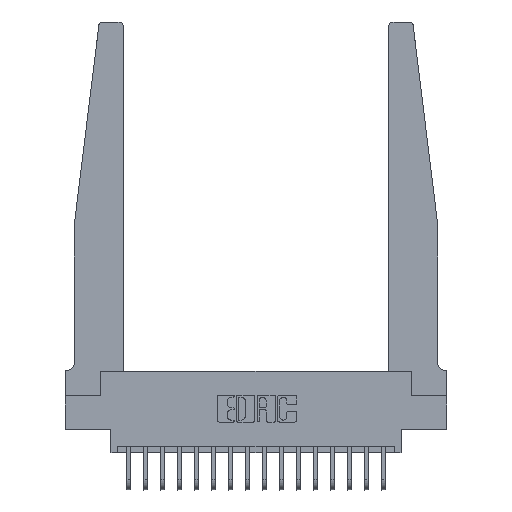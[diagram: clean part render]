
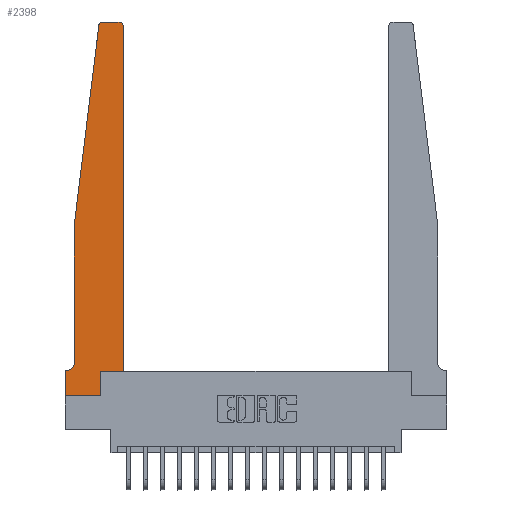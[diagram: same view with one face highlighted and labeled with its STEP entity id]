
A CAD part, top view. The second image highlights one B-rep face of the part: STEP entity #2398.
In plain terms, the highlighted planar face has unit normal (0, 0, 1).
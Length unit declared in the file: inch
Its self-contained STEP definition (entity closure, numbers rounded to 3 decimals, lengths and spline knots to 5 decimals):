
#23 = VECTOR ( 'NONE', #3496, 39.37008 ) ;
#395 = VERTEX_POINT ( 'NONE', #11442 ) ;
#416 = LINE ( 'NONE', #11971, #4247 ) ;
#700 = CARTESIAN_POINT ( 'NONE',  ( 0., 0.1875, 0.37 ) ) ;
#761 = CARTESIAN_POINT ( 'NONE',  ( 0.065, 0.2375, 0.37 ) ) ;
#1073 = AXIS2_PLACEMENT_3D ( 'NONE', #1193, #7030, #4144 ) ;
#1103 = VECTOR ( 'NONE', #1638, 39.37008 ) ;
#1130 = ORIENTED_EDGE ( 'NONE', *, *, #9392, .T. ) ;
#1193 = CARTESIAN_POINT ( 'NONE',  ( 0.395, 2.72, 0.37 ) ) ;
#1266 = VERTEX_POINT ( 'NONE', #8706 ) ;
#1410 = DIRECTION ( 'NONE',  ( 1., 0., 0. ) ) ;
#1638 = DIRECTION ( 'NONE',  ( 0., 1., 0. ) ) ;
#1659 = EDGE_CURVE ( 'NONE', #17871, #16791, #14069, .T. ) ;
#1807 = EDGE_CURVE ( 'NONE', #6830, #1266, #15064, .T. ) ;
#2285 = LINE ( 'NONE', #8151, #11412 ) ;
#2296 = FACE_OUTER_BOUND ( 'NONE', #10559, .T. ) ;
#2398 = ADVANCED_FACE ( 'NONE', ( #2296 ), #6512, .T. ) ;
#2771 = ORIENTED_EDGE ( 'NONE', *, *, #8517, .T. ) ;
#2815 = CARTESIAN_POINT ( 'NONE',  ( 0.2605, 0., 0.37 ) ) ;
#3151 = DIRECTION ( 'NONE',  ( 0., 1., 0. ) ) ;
#3366 = CARTESIAN_POINT ( 'NONE',  ( 0., 0.1875, 0.37 ) ) ;
#3496 = DIRECTION ( 'NONE',  ( 0., -1., 0. ) ) ;
#3754 = DIRECTION ( 'NONE',  ( 1., 0., 0. ) ) ;
#3782 = VECTOR ( 'NONE', #3754, 39.37008 ) ;
#3807 = ORIENTED_EDGE ( 'NONE', *, *, #1659, .T. ) ;
#3836 = VECTOR ( 'NONE', #13923, 39.37008 ) ;
#3914 = ORIENTED_EDGE ( 'NONE', *, *, #5635, .T. ) ;
#3952 = CARTESIAN_POINT ( 'NONE',  ( 0.425, 0.18, 0.37 ) ) ;
#4144 = DIRECTION ( 'NONE',  ( 1., 0., 0. ) ) ;
#4247 = VECTOR ( 'NONE', #17502, 39.37008 ) ;
#4494 = VERTEX_POINT ( 'NONE', #15113 ) ;
#4569 = CARTESIAN_POINT ( 'NONE',  ( 0.015, 0.2375, 0.37 ) ) ;
#4666 = DIRECTION ( 'NONE',  ( 0., 0., -1. ) ) ;
#4857 = CARTESIAN_POINT ( 'NONE',  ( 0.395, 2.75, 0.37 ) ) ;
#5635 = EDGE_CURVE ( 'NONE', #17623, #395, #10920, .T. ) ;
#5710 = ORIENTED_EDGE ( 'NONE', *, *, #17964, .T. ) ;
#5864 = ORIENTED_EDGE ( 'NONE', *, *, #12628, .T. ) ;
#6148 = VERTEX_POINT ( 'NONE', #17131 ) ;
#6265 = CIRCLE ( 'NONE', #1073, 0.03 ) ;
#6512 = PLANE ( 'NONE',  #12180 ) ;
#6687 = DIRECTION ( 'NONE',  ( -1., 0., 0. ) ) ;
#6830 = VERTEX_POINT ( 'NONE', #700 ) ;
#7030 = DIRECTION ( 'NONE',  ( 0., 0., 1. ) ) ;
#7727 = DIRECTION ( 'NONE',  ( -1., 0., 0. ) ) ;
#7772 = CARTESIAN_POINT ( 'NONE',  ( 0.25, 2.75, 0.37 ) ) ;
#7882 = DIRECTION ( 'NONE',  ( 0., -1., 0. ) ) ;
#8151 = CARTESIAN_POINT ( 'NONE',  ( 0.065, 0.1875, 0.37 ) ) ;
#8205 = LINE ( 'NONE', #3952, #3782 ) ;
#8338 = VERTEX_POINT ( 'NONE', #15226 ) ;
#8358 = CARTESIAN_POINT ( 'NONE',  ( 0., 0., 0.37 ) ) ;
#8517 = EDGE_CURVE ( 'NONE', #4494, #6830, #2285, .T. ) ;
#8706 = CARTESIAN_POINT ( 'NONE',  ( 0., 0., 0.37 ) ) ;
#8928 = LINE ( 'NONE', #10393, #15986 ) ;
#9020 = CARTESIAN_POINT ( 'NONE',  ( 0.425, 0.18, 0.37 ) ) ;
#9392 = EDGE_CURVE ( 'NONE', #6148, #17055, #6265, .T. ) ;
#9807 = CARTESIAN_POINT ( 'NONE',  ( 0.425, 0.18, 0.37 ) ) ;
#10034 = CIRCLE ( 'NONE', #17343, 0.05 ) ;
#10393 = CARTESIAN_POINT ( 'NONE',  ( 0.2605, 0.18, 0.37 ) ) ;
#10559 = EDGE_LOOP ( 'NONE', ( #5864, #3914, #5710, #3807, #15514, #2771, #14282, #18601, #13745, #17992, #18495, #1130 ) ) ;
#10567 = EDGE_CURVE ( 'NONE', #8338, #13510, #8205, .T. ) ;
#10920 = CIRCLE ( 'NONE', #16694, 0.03 ) ;
#11155 = VERTEX_POINT ( 'NONE', #2815 ) ;
#11381 = EDGE_CURVE ( 'NONE', #11155, #8338, #8928, .T. ) ;
#11412 = VECTOR ( 'NONE', #6687, 39.37008 ) ;
#11442 = CARTESIAN_POINT ( 'NONE',  ( 0.24675, 2.72367, 0.37 ) ) ;
#11971 = CARTESIAN_POINT ( 'NONE',  ( 0.065, 1.25, 0.37 ) ) ;
#12180 = AXIS2_PLACEMENT_3D ( 'NONE', #3366, #15053, #17182 ) ;
#12628 = EDGE_CURVE ( 'NONE', #17055, #17623, #13826, .T. ) ;
#12774 = EDGE_CURVE ( 'NONE', #1266, #11155, #15507, .T. ) ;
#12801 = EDGE_CURVE ( 'NONE', #13510, #6148, #13264, .T. ) ;
#12914 = CARTESIAN_POINT ( 'NONE',  ( 0.065, 1.25, 0.37 ) ) ;
#13001 = VECTOR ( 'NONE', #14278, 39.37008 ) ;
#13264 = LINE ( 'NONE', #9020, #1103 ) ;
#13510 = VERTEX_POINT ( 'NONE', #9807 ) ;
#13745 = ORIENTED_EDGE ( 'NONE', *, *, #11381, .T. ) ;
#13748 = CARTESIAN_POINT ( 'NONE',  ( 0., 0., 0.37 ) ) ;
#13826 = LINE ( 'NONE', #7772, #3836 ) ;
#13923 = DIRECTION ( 'NONE',  ( -1., 0., 0. ) ) ;
#14069 = LINE ( 'NONE', #18390, #23 ) ;
#14161 = CARTESIAN_POINT ( 'NONE',  ( 0.27653, 2.72, 0.37 ) ) ;
#14278 = DIRECTION ( 'NONE',  ( 1., 0., 0. ) ) ;
#14282 = ORIENTED_EDGE ( 'NONE', *, *, #1807, .T. ) ;
#15053 = DIRECTION ( 'NONE',  ( 0., 0., 1. ) ) ;
#15064 = LINE ( 'NONE', #13748, #15227 ) ;
#15113 = CARTESIAN_POINT ( 'NONE',  ( 0.015, 0.1875, 0.37 ) ) ;
#15226 = CARTESIAN_POINT ( 'NONE',  ( 0.2605, 0.18, 0.37 ) ) ;
#15227 = VECTOR ( 'NONE', #7882, 39.37008 ) ;
#15507 = LINE ( 'NONE', #8358, #13001 ) ;
#15514 = ORIENTED_EDGE ( 'NONE', *, *, #15799, .T. ) ;
#15799 = EDGE_CURVE ( 'NONE', #16791, #4494, #10034, .T. ) ;
#15986 = VECTOR ( 'NONE', #3151, 39.37008 ) ;
#16694 = AXIS2_PLACEMENT_3D ( 'NONE', #14161, #18585, #1410 ) ;
#16791 = VERTEX_POINT ( 'NONE', #761 ) ;
#17055 = VERTEX_POINT ( 'NONE', #4857 ) ;
#17131 = CARTESIAN_POINT ( 'NONE',  ( 0.425, 2.72, 0.37 ) ) ;
#17182 = DIRECTION ( 'NONE',  ( 1., 0., 0. ) ) ;
#17343 = AXIS2_PLACEMENT_3D ( 'NONE', #4569, #4666, #7727 ) ;
#17502 = DIRECTION ( 'NONE',  ( -0.122, -0.992, 0. ) ) ;
#17623 = VERTEX_POINT ( 'NONE', #18365 ) ;
#17871 = VERTEX_POINT ( 'NONE', #12914 ) ;
#17964 = EDGE_CURVE ( 'NONE', #395, #17871, #416, .T. ) ;
#17992 = ORIENTED_EDGE ( 'NONE', *, *, #10567, .T. ) ;
#18365 = CARTESIAN_POINT ( 'NONE',  ( 0.27653, 2.75, 0.37 ) ) ;
#18390 = CARTESIAN_POINT ( 'NONE',  ( 0.065, 1.25, 0.37 ) ) ;
#18495 = ORIENTED_EDGE ( 'NONE', *, *, #12801, .T. ) ;
#18585 = DIRECTION ( 'NONE',  ( 0., 0., 1. ) ) ;
#18601 = ORIENTED_EDGE ( 'NONE', *, *, #12774, .T. ) ;
